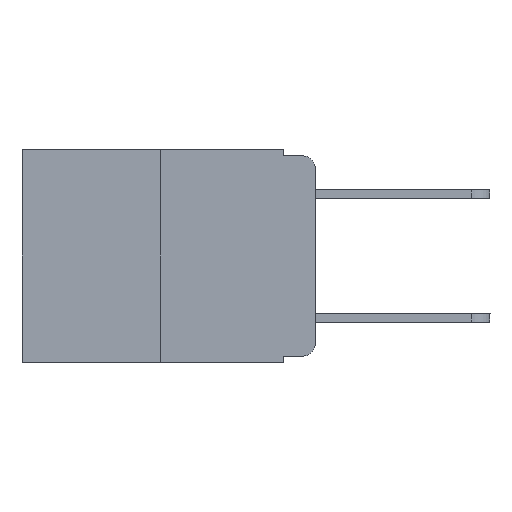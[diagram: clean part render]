
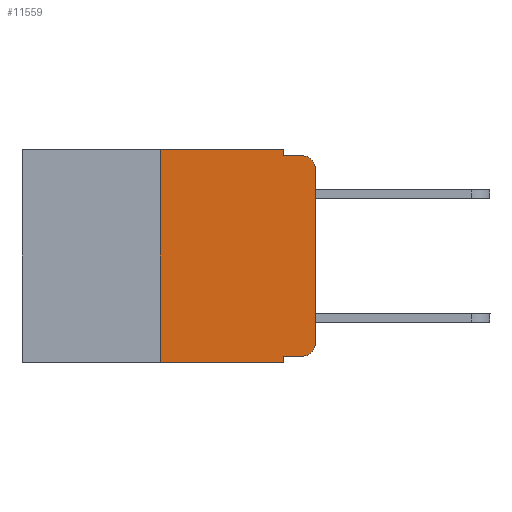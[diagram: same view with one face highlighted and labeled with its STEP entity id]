
A CAD part, left-side view. The second image highlights one B-rep face of the part: STEP entity #11559.
In plain terms, the highlighted planar face has unit normal (-1, 0, 0).
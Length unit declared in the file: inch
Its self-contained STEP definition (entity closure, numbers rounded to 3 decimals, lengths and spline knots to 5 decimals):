
#371 = DIRECTION ( 'NONE',  ( -1., 0., 0. ) ) ;
#502 = DIRECTION ( 'NONE',  ( 0., 0., -1. ) ) ;
#764 = CARTESIAN_POINT ( 'NONE',  ( 0., 0.25, 0. ) ) ;
#994 = DIRECTION ( 'NONE',  ( 0., -1., 0. ) ) ;
#1204 = DIRECTION ( 'NONE',  ( 0., 0., 1. ) ) ;
#1214 = ORIENTED_EDGE ( 'NONE', *, *, #11601, .T. ) ;
#1714 = EDGE_CURVE ( 'NONE', #2598, #4740, #10490, .T. ) ;
#1745 = CARTESIAN_POINT ( 'NONE',  ( 0., 0.473, -0.343 ) ) ;
#1881 = FACE_OUTER_BOUND ( 'NONE', #10867, .T. ) ;
#1915 = VECTOR ( 'NONE', #10513, 39.37008 ) ;
#1993 = AXIS2_PLACEMENT_3D ( 'NONE', #2983, #14664, #16014 ) ;
#2142 = EDGE_CURVE ( 'NONE', #7372, #15072, #11509, .T. ) ;
#2257 = EDGE_CURVE ( 'NONE', #15406, #12619, #16501, .T. ) ;
#2598 = VERTEX_POINT ( 'NONE', #12569 ) ;
#2882 = CARTESIAN_POINT ( 'NONE',  ( 0., 0.051, -0.333 ) ) ;
#2983 = CARTESIAN_POINT ( 'NONE',  ( 0., 0.473, 0. ) ) ;
#3305 = LINE ( 'NONE', #16507, #16720 ) ;
#4408 = CIRCLE ( 'NONE', #13435, 0.02 ) ;
#4413 = DIRECTION ( 'NONE',  ( -1., 0., 0. ) ) ;
#4740 = VERTEX_POINT ( 'NONE', #764 ) ;
#4862 = EDGE_CURVE ( 'NONE', #4740, #16231, #13506, .T. ) ;
#5149 = EDGE_CURVE ( 'NONE', #16231, #15406, #12669, .T. ) ;
#5166 = ORIENTED_EDGE ( 'NONE', *, *, #2257, .F. ) ;
#5519 = ORIENTED_EDGE ( 'NONE', *, *, #15138, .T. ) ;
#5621 = CARTESIAN_POINT ( 'NONE',  ( 0., 0.02, -0.313 ) ) ;
#6415 = VECTOR ( 'NONE', #8167, 39.37008 ) ;
#6418 = LINE ( 'NONE', #1745, #11306 ) ;
#6429 = AXIS2_PLACEMENT_3D ( 'NONE', #9307, #4413, #502 ) ;
#6477 = CARTESIAN_POINT ( 'NONE',  ( 0., 0.051, 0. ) ) ;
#6761 = ORIENTED_EDGE ( 'NONE', *, *, #10886, .F. ) ;
#6949 = VECTOR ( 'NONE', #994, 39.37008 ) ;
#7223 = CARTESIAN_POINT ( 'NONE',  ( 0., 0.02, -0.333 ) ) ;
#7346 = DIRECTION ( 'NONE',  ( 0., 0., 1. ) ) ;
#7347 = VECTOR ( 'NONE', #10742, 39.37008 ) ;
#7372 = VERTEX_POINT ( 'NONE', #12380 ) ;
#7411 = CARTESIAN_POINT ( 'NONE',  ( 0., 0., -0.313 ) ) ;
#7922 = ORIENTED_EDGE ( 'NONE', *, *, #2142, .T. ) ;
#8000 = ORIENTED_EDGE ( 'NONE', *, *, #5149, .F. ) ;
#8167 = DIRECTION ( 'NONE',  ( 0., -1., 0. ) ) ;
#8246 = DIRECTION ( 'NONE',  ( 0., -1., 0. ) ) ;
#8658 = ORIENTED_EDGE ( 'NONE', *, *, #10269, .T. ) ;
#8703 = CIRCLE ( 'NONE', #6429, 0.02 ) ;
#9307 = CARTESIAN_POINT ( 'NONE',  ( 0., 0.02, -0.03 ) ) ;
#9463 = VECTOR ( 'NONE', #16075, 39.37008 ) ;
#9518 = DIRECTION ( 'NONE',  ( 0., 0., -1. ) ) ;
#10013 = CARTESIAN_POINT ( 'NONE',  ( 0., 0.473, 0. ) ) ;
#10269 = EDGE_CURVE ( 'NONE', #15072, #16109, #4408, .T. ) ;
#10490 = LINE ( 'NONE', #12932, #11526 ) ;
#10513 = DIRECTION ( 'NONE',  ( 0., 0., -1. ) ) ;
#10692 = CARTESIAN_POINT ( 'NONE',  ( 0., 0.051, -0.343 ) ) ;
#10742 = DIRECTION ( 'NONE',  ( 0., 0., -1. ) ) ;
#10867 = EDGE_LOOP ( 'NONE', ( #5519, #1214, #5166, #8000, #11239, #14257, #14351, #6761, #7922, #8658 ) ) ;
#10886 = EDGE_CURVE ( 'NONE', #7372, #12727, #12611, .T. ) ;
#11239 = ORIENTED_EDGE ( 'NONE', *, *, #4862, .F. ) ;
#11306 = VECTOR ( 'NONE', #8246, 39.37008 ) ;
#11509 = LINE ( 'NONE', #2882, #6415 ) ;
#11526 = VECTOR ( 'NONE', #1204, 39.37008 ) ;
#11559 = ADVANCED_FACE ( 'NONE', ( #1881 ), #11936, .F. ) ;
#11601 = EDGE_CURVE ( 'NONE', #12135, #12619, #8703, .T. ) ;
#11747 = CARTESIAN_POINT ( 'NONE',  ( 0., 0., -0.03 ) ) ;
#11936 = PLANE ( 'NONE',  #1993 ) ;
#12135 = VERTEX_POINT ( 'NONE', #11747 ) ;
#12195 = EDGE_CURVE ( 'NONE', #2598, #12727, #6418, .T. ) ;
#12380 = CARTESIAN_POINT ( 'NONE',  ( 0., 0.051, -0.333 ) ) ;
#12569 = CARTESIAN_POINT ( 'NONE',  ( 0., 0.25, -0.343 ) ) ;
#12611 = LINE ( 'NONE', #14688, #1915 ) ;
#12619 = VERTEX_POINT ( 'NONE', #17017 ) ;
#12669 = LINE ( 'NONE', #13400, #7347 ) ;
#12727 = VERTEX_POINT ( 'NONE', #10692 ) ;
#12932 = CARTESIAN_POINT ( 'NONE',  ( 0., 0.25, 0. ) ) ;
#13400 = CARTESIAN_POINT ( 'NONE',  ( 0., 0.051, 0. ) ) ;
#13408 = CARTESIAN_POINT ( 'NONE',  ( 0., 0.051, -0.01 ) ) ;
#13435 = AXIS2_PLACEMENT_3D ( 'NONE', #5621, #371, #9518 ) ;
#13506 = LINE ( 'NONE', #10013, #6949 ) ;
#14257 = ORIENTED_EDGE ( 'NONE', *, *, #1714, .F. ) ;
#14351 = ORIENTED_EDGE ( 'NONE', *, *, #12195, .T. ) ;
#14664 = DIRECTION ( 'NONE',  ( 1., 0., 0. ) ) ;
#14688 = CARTESIAN_POINT ( 'NONE',  ( 0., 0.051, 0. ) ) ;
#15072 = VERTEX_POINT ( 'NONE', #7223 ) ;
#15138 = EDGE_CURVE ( 'NONE', #16109, #12135, #3305, .T. ) ;
#15406 = VERTEX_POINT ( 'NONE', #16843 ) ;
#16014 = DIRECTION ( 'NONE',  ( 0., 0., -1. ) ) ;
#16075 = DIRECTION ( 'NONE',  ( 0., -1., 0. ) ) ;
#16109 = VERTEX_POINT ( 'NONE', #7411 ) ;
#16231 = VERTEX_POINT ( 'NONE', #6477 ) ;
#16501 = LINE ( 'NONE', #13408, #9463 ) ;
#16507 = CARTESIAN_POINT ( 'NONE',  ( 0., 0., 0. ) ) ;
#16720 = VECTOR ( 'NONE', #7346, 39.37008 ) ;
#16843 = CARTESIAN_POINT ( 'NONE',  ( 0., 0.051, -0.01 ) ) ;
#17017 = CARTESIAN_POINT ( 'NONE',  ( 0., 0.02, -0.01 ) ) ;
